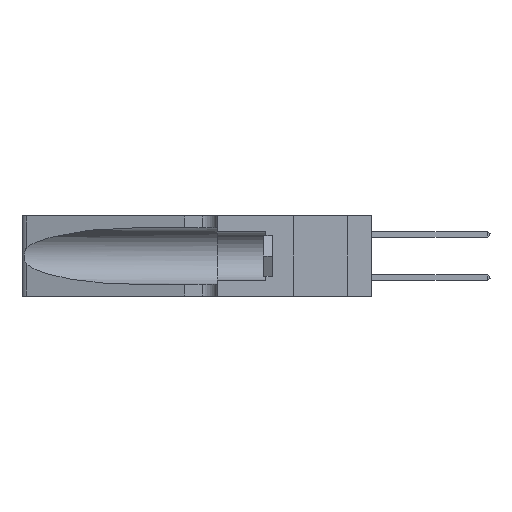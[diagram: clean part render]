
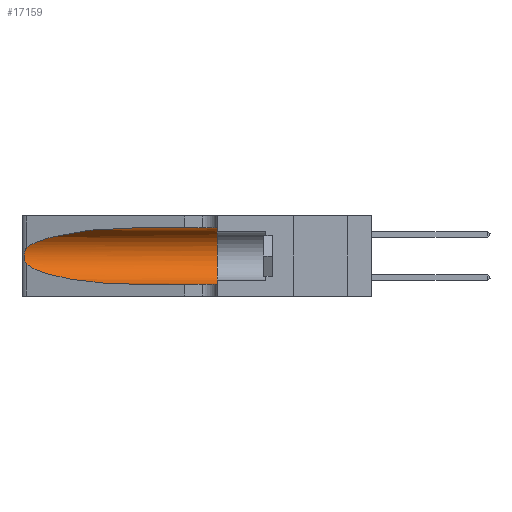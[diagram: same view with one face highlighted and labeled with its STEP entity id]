
A CAD part, left-side view. The second image highlights one B-rep face of the part: STEP entity #17159.
In plain terms, the highlighted cylindrical face has radius 3.308 mm (diameter 6.617 mm), a partial arc.
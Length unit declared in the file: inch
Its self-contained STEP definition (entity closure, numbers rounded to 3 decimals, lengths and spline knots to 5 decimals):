
#327 = VERTEX_POINT ( 'NONE', #23027 ) ;
#471 = EDGE_CURVE ( 'NONE', #327, #16663, #9910, .T. ) ;
#1173 = ORIENTED_EDGE ( 'NONE', *, *, #2636, .T. ) ;
#1838 = DIRECTION ( 'NONE',  ( 0., 1., 0. ) ) ;
#2435 = CARTESIAN_POINT ( 'NONE',  ( 0.25639, 1.23184, 0.21858 ) ) ;
#2636 = EDGE_CURVE ( 'NONE', #27094, #19061, #23096, .T. ) ;
#3700 = CARTESIAN_POINT ( 'NONE',  ( 0.25487, 1.22718, 0.14631 ) ) ;
#3827 = ORIENTED_EDGE ( 'NONE', *, *, #17252, .F. ) ;
#4057 = CARTESIAN_POINT ( 'NONE',  ( 0.18966, 0.96281, 0.31525 ) ) ;
#4086 = CARTESIAN_POINT ( 'NONE',  ( 0.1305, 0.35, 0.31525 ) ) ;
#4382 = ORIENTED_EDGE ( 'NONE', *, *, #12928, .T. ) ;
#6084 = CARTESIAN_POINT ( 'NONE',  ( 0.1305, 0.35, 0.05475 ) ) ;
#6169 = EDGE_LOOP ( 'NONE', ( #8777, #20610, #4382, #1173, #17274, #3827 ) ) ;
#6812 = CARTESIAN_POINT ( 'NONE',  ( 0.25487, 1.22718, 0.22369 ) ) ;
#6939 = DIRECTION ( 'NONE',  ( 0., -1., 0. ) ) ;
#7539 = CARTESIAN_POINT ( 'NONE',  ( 0.25555, 1.22993, 0.14849 ) ) ;
#8604 = CARTESIAN_POINT ( 'NONE',  ( 0.18966, 0.96281, 0.05475 ) ) ;
#8777 = ORIENTED_EDGE ( 'NONE', *, *, #16443, .T. ) ;
#8858 = CARTESIAN_POINT ( 'NONE',  ( 0.2373, 1.15595, 0.28018 ) ) ;
#9817 = CARTESIAN_POINT ( 'NONE',  ( 0.25789, 1.23486, 0.15765 ) ) ;
#9823 = CARTESIAN_POINT ( 'NONE',  ( 0.1305, 0.72297, 0.31525 ) ) ;
#9910 = B_SPLINE_CURVE_WITH_KNOTS ( 'NONE', 3,
 ( #6812, #24018, #2435, #18836, #20857, #21030, #23148, #23221, #27714, #25404, #9817, #23119, #7539, #20933 ),
 .UNSPECIFIED., .F., .F.,
 ( 4, 2, 2, 2, 2, 2, 4 ),
 ( 0., 0.00027, 0.00053, 0.00107, 0.0016, 0.00187, 0.00214 ),
 .UNSPECIFIED. ) ;
#10425 = VERTEX_POINT ( 'NONE', #9823 ) ;
#10913 = CYLINDRICAL_SURFACE ( 'NONE', #13043, 0.13025 ) ;
#11392 = CARTESIAN_POINT ( 'NONE',  ( 0.1305, 0.72297, 0.05475 ) ) ;
#11577 = VECTOR ( 'NONE', #24724, 39.37008 ) ;
#12928 = EDGE_CURVE ( 'NONE', #16663, #27094, #19988, .T. ) ;
#13043 = AXIS2_PLACEMENT_3D ( 'NONE', #20462, #18172, #22751 ) ;
#14330 = EDGE_CURVE ( 'NONE', #17781, #19061, #22040, .T. ) ;
#14921 = LINE ( 'NONE', #27628, #20286 ) ;
#15991 = CARTESIAN_POINT ( 'NONE',  ( 0.1305, 0.35, 0.185 ) ) ;
#16443 = EDGE_CURVE ( 'NONE', #10425, #327, #20786, .T. ) ;
#16663 = VERTEX_POINT ( 'NONE', #16984 ) ;
#16984 = CARTESIAN_POINT ( 'NONE',  ( 0.25487, 1.22718, 0.14631 ) ) ;
#17159 = ADVANCED_FACE ( 'NONE', ( #29905 ), #10913, .F. ) ;
#17252 = EDGE_CURVE ( 'NONE', #10425, #17781, #14921, .T. ) ;
#17274 = ORIENTED_EDGE ( 'NONE', *, *, #14330, .F. ) ;
#17781 = VERTEX_POINT ( 'NONE', #4086 ) ;
#18172 = DIRECTION ( 'NONE',  ( 0., -1., 0. ) ) ;
#18297 = DIRECTION ( 'NONE',  ( 0., 0., 1. ) ) ;
#18836 = CARTESIAN_POINT ( 'NONE',  ( 0.25787, 1.23484, 0.2124 ) ) ;
#19061 = VERTEX_POINT ( 'NONE', #6084 ) ;
#19988 =( BOUNDED_CURVE ( )  B_SPLINE_CURVE ( 3, ( #3700, #20145, #8604, #24733 ),
 .UNSPECIFIED., .F., .F. ) 
 B_SPLINE_CURVE_WITH_KNOTS ( ( 4, 4 ),
 ( 3.44316, 4.71239 ),
 .UNSPECIFIED. ) 
 CURVE ( )  GEOMETRIC_REPRESENTATION_ITEM ( )  RATIONAL_B_SPLINE_CURVE ( ( 1., 0.87, 0.87, 1. ) ) 
 REPRESENTATION_ITEM ( '' )  );
#20145 = CARTESIAN_POINT ( 'NONE',  ( 0.2373, 1.15595, 0.08982 ) ) ;
#20286 = VECTOR ( 'NONE', #6939, 39.37008 ) ;
#20371 = AXIS2_PLACEMENT_3D ( 'NONE', #15991, #1838, #18297 ) ;
#20393 = CARTESIAN_POINT ( 'NONE',  ( 0.1305, 0.72297, 0.31525 ) ) ;
#20462 = CARTESIAN_POINT ( 'NONE',  ( 0.1305, 1.61858, 0.185 ) ) ;
#20610 = ORIENTED_EDGE ( 'NONE', *, *, #471, .T. ) ;
#20786 =( BOUNDED_CURVE ( )  B_SPLINE_CURVE ( 3, ( #20393, #4057, #8858, #24971 ),
 .UNSPECIFIED., .F., .T. ) 
 B_SPLINE_CURVE_WITH_KNOTS ( ( 4, 4 ),
 ( 1.5708, 2.84003 ),
 .UNSPECIFIED. ) 
 CURVE ( )  GEOMETRIC_REPRESENTATION_ITEM ( )  RATIONAL_B_SPLINE_CURVE ( ( 1., 0.87, 0.87, 1. ) ) 
 REPRESENTATION_ITEM ( '' )  );
#20857 = CARTESIAN_POINT ( 'NONE',  ( 0.25854, 1.2359, 0.20912 ) ) ;
#20933 = CARTESIAN_POINT ( 'NONE',  ( 0.25487, 1.22718, 0.14631 ) ) ;
#21030 = CARTESIAN_POINT ( 'NONE',  ( 0.26018, 1.23835, 0.19895 ) ) ;
#22040 = CIRCLE ( 'NONE', #20371, 0.13025 ) ;
#22751 = DIRECTION ( 'NONE',  ( 0., 0., -1. ) ) ;
#23027 = CARTESIAN_POINT ( 'NONE',  ( 0.25487, 1.22718, 0.22369 ) ) ;
#23096 = LINE ( 'NONE', #28076, #11577 ) ;
#23119 = CARTESIAN_POINT ( 'NONE',  ( 0.25639, 1.23186, 0.15144 ) ) ;
#23148 = CARTESIAN_POINT ( 'NONE',  ( 0.26075, 1.23896, 0.19203 ) ) ;
#23221 = CARTESIAN_POINT ( 'NONE',  ( 0.26075, 1.23896, 0.178 ) ) ;
#24018 = CARTESIAN_POINT ( 'NONE',  ( 0.25555, 1.22994, 0.2215 ) ) ;
#24724 = DIRECTION ( 'NONE',  ( 0., -1., 0. ) ) ;
#24733 = CARTESIAN_POINT ( 'NONE',  ( 0.1305, 0.72297, 0.05475 ) ) ;
#24971 = CARTESIAN_POINT ( 'NONE',  ( 0.25487, 1.22718, 0.22369 ) ) ;
#25404 = CARTESIAN_POINT ( 'NONE',  ( 0.25856, 1.23593, 0.16098 ) ) ;
#27094 = VERTEX_POINT ( 'NONE', #11392 ) ;
#27628 = CARTESIAN_POINT ( 'NONE',  ( 0.1305, 1.61858, 0.31525 ) ) ;
#27714 = CARTESIAN_POINT ( 'NONE',  ( 0.26017, 1.23833, 0.17102 ) ) ;
#28076 = CARTESIAN_POINT ( 'NONE',  ( 0.1305, 1.61858, 0.05475 ) ) ;
#29905 = FACE_OUTER_BOUND ( 'NONE', #6169, .T. ) ;
